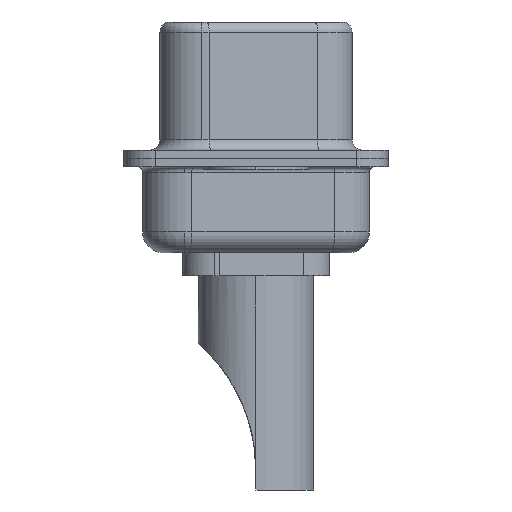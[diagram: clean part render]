
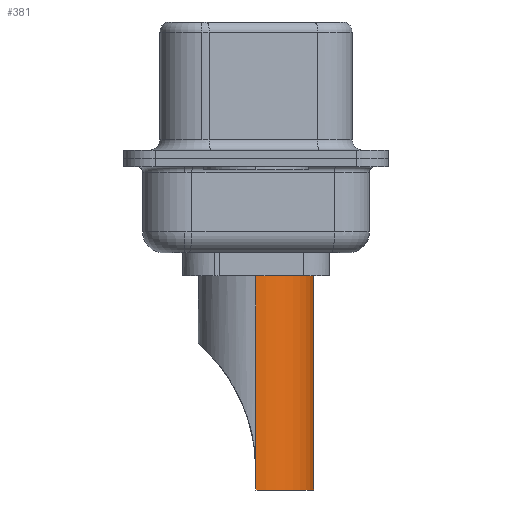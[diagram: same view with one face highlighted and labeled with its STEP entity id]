
A CAD part, left-side view. The second image highlights one B-rep face of the part: STEP entity #381.
In plain terms, the highlighted cylindrical face has radius 2.75 mm (diameter 5.5 mm), a partial arc.
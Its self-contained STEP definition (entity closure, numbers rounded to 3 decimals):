
#350 = CIRCLE ( 'NONE', #7880, 2.75 ) ;
#381 = ADVANCED_FACE ( 'NONE', ( #9845 ), #1735, .T. ) ;
#400 = VERTEX_POINT ( 'NONE', #3917 ) ;
#470 = EDGE_CURVE ( 'NONE', #400, #1988, #8598, .T. ) ;
#494 = ORIENTED_EDGE ( 'NONE', *, *, #4000, .F. ) ;
#501 = CARTESIAN_POINT ( 'NONE',  ( 2.75, 0., 4.234 ) ) ;
#747 = EDGE_CURVE ( 'NONE', #982, #8471, #350, .T. ) ;
#778 = DIRECTION ( 'NONE',  ( 0., 0., 1. ) ) ;
#810 = EDGE_CURVE ( 'NONE', #1752, #982, #6747, .T. ) ;
#982 = VERTEX_POINT ( 'NONE', #4644 ) ;
#1534 = CARTESIAN_POINT ( 'NONE',  ( 2.75, 0., -8.7 ) ) ;
#1735 = CYLINDRICAL_SURFACE ( 'NONE', #7231, 2.75 ) ;
#1752 = VERTEX_POINT ( 'NONE', #2113 ) ;
#1988 = VERTEX_POINT ( 'NONE', #7883 ) ;
#2113 = CARTESIAN_POINT ( 'NONE',  ( -2.75, 0., -7.764 ) ) ;
#2219 = DIRECTION ( 'NONE',  ( 0., 0., 1. ) ) ;
#2639 = DIRECTION ( 'NONE',  ( 0., 0., 1. ) ) ;
#2995 = DIRECTION ( 'NONE',  ( 0., 0., -1. ) ) ;
#3118 = ORIENTED_EDGE ( 'NONE', *, *, #3957, .F. ) ;
#3214 = DIRECTION ( 'NONE',  ( 0., 0., -1. ) ) ;
#3217 = ORIENTED_EDGE ( 'NONE', *, *, #747, .T. ) ;
#3917 = CARTESIAN_POINT ( 'NONE',  ( 2.75, 0., -7.764 ) ) ;
#3957 = EDGE_CURVE ( 'NONE', #400, #8471, #7785, .T. ) ;
#4000 = EDGE_CURVE ( 'NONE', #4799, #1988, #4677, .T. ) ;
#4445 = LINE ( 'NONE', #12445, #11430 ) ;
#4644 = CARTESIAN_POINT ( 'NONE',  ( -2.75, 0., -8.7 ) ) ;
#4677 = CIRCLE ( 'NONE', #6721, 2.75 ) ;
#4799 = VERTEX_POINT ( 'NONE', #5353 ) ;
#5248 = ORIENTED_EDGE ( 'NONE', *, *, #470, .T. ) ;
#5353 = CARTESIAN_POINT ( 'NONE',  ( -2.75, 0., 1.5 ) ) ;
#5454 = CARTESIAN_POINT ( 'NONE',  ( 0., 0., -8.7 ) ) ;
#5562 = VECTOR ( 'NONE', #3214, 1000. ) ;
#6141 = DIRECTION ( 'NONE',  ( 1., 0., 0. ) ) ;
#6437 = ORIENTED_EDGE ( 'NONE', *, *, #810, .T. ) ;
#6721 = AXIS2_PLACEMENT_3D ( 'NONE', #8840, #2219, #6141 ) ;
#6747 = LINE ( 'NONE', #12482, #9049 ) ;
#7231 = AXIS2_PLACEMENT_3D ( 'NONE', #10796, #2639, #11582 ) ;
#7785 = LINE ( 'NONE', #11575, #5562 ) ;
#7880 = AXIS2_PLACEMENT_3D ( 'NONE', #5454, #8557, #11188 ) ;
#7883 = CARTESIAN_POINT ( 'NONE',  ( 2.75, 0., 1.5 ) ) ;
#8471 = VERTEX_POINT ( 'NONE', #1534 ) ;
#8557 = DIRECTION ( 'NONE',  ( 0., 0., 1. ) ) ;
#8598 = LINE ( 'NONE', #501, #10876 ) ;
#8840 = CARTESIAN_POINT ( 'NONE',  ( 0., 0., 1.5 ) ) ;
#9049 = VECTOR ( 'NONE', #2995, 1000. ) ;
#9488 = EDGE_CURVE ( 'NONE', #1752, #4799, #4445, .T. ) ;
#9845 = FACE_OUTER_BOUND ( 'NONE', #10992, .T. ) ;
#10796 = CARTESIAN_POINT ( 'NONE',  ( 0., 0., 4.234 ) ) ;
#10876 = VECTOR ( 'NONE', #11732, 1000. ) ;
#10992 = EDGE_LOOP ( 'NONE', ( #12465, #6437, #3217, #3118, #5248, #494 ) ) ;
#11188 = DIRECTION ( 'NONE',  ( 1., 0., 0. ) ) ;
#11430 = VECTOR ( 'NONE', #778, 1000. ) ;
#11575 = CARTESIAN_POINT ( 'NONE',  ( 2.75, 0., -8.7 ) ) ;
#11582 = DIRECTION ( 'NONE',  ( 1., 0., 0. ) ) ;
#11732 = DIRECTION ( 'NONE',  ( 0., 0., 1. ) ) ;
#12445 = CARTESIAN_POINT ( 'NONE',  ( -2.75, 0., 4.234 ) ) ;
#12465 = ORIENTED_EDGE ( 'NONE', *, *, #9488, .F. ) ;
#12482 = CARTESIAN_POINT ( 'NONE',  ( -2.75, 0., -8.7 ) ) ;
